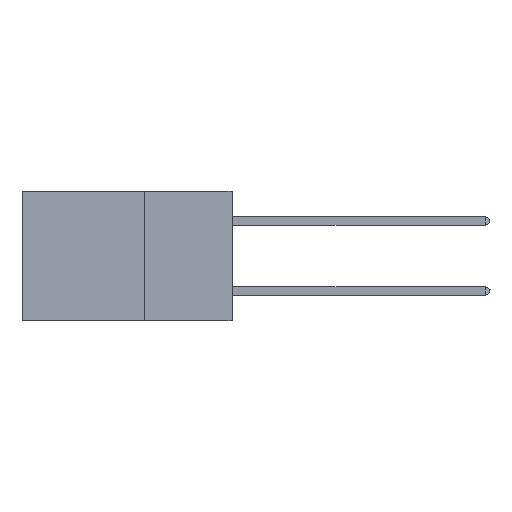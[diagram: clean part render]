
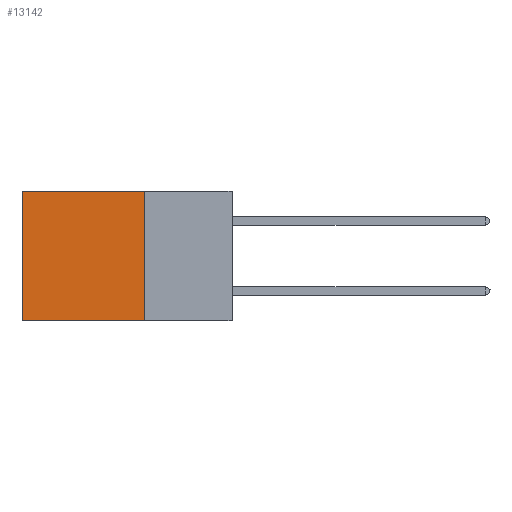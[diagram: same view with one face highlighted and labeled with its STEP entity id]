
A CAD part, left-side view. The second image highlights one B-rep face of the part: STEP entity #13142.
In plain terms, the highlighted planar face has unit normal (-1, 0, 0).
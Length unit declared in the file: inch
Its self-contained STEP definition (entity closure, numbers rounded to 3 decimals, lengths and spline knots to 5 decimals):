
#120 = CARTESIAN_POINT ( 'NONE',  ( 0.2875, 0.25, 0. ) ) ;
#332 = CARTESIAN_POINT ( 'NONE',  ( 0.2875, 0.25, -0.37 ) ) ;
#956 = ORIENTED_EDGE ( 'NONE', *, *, #16880, .F. ) ;
#1086 = VERTEX_POINT ( 'NONE', #6090 ) ;
#1681 = DIRECTION ( 'NONE',  ( 0., 1., 0. ) ) ;
#1749 = LINE ( 'NONE', #332, #8444 ) ;
#2374 = ORIENTED_EDGE ( 'NONE', *, *, #4101, .F. ) ;
#2925 = EDGE_LOOP ( 'NONE', ( #8994, #2374, #956, #4639 ) ) ;
#3289 = LINE ( 'NONE', #3307, #4132 ) ;
#3307 = CARTESIAN_POINT ( 'NONE',  ( 0.2875, 0.6, 0. ) ) ;
#3904 = PLANE ( 'NONE',  #5573 ) ;
#4068 = CARTESIAN_POINT ( 'NONE',  ( 0.2875, 0.6, 0. ) ) ;
#4101 = EDGE_CURVE ( 'NONE', #8331, #1086, #1749, .T. ) ;
#4132 = VECTOR ( 'NONE', #11289, 39.37008 ) ;
#4258 = VECTOR ( 'NONE', #8381, 39.37008 ) ;
#4639 = ORIENTED_EDGE ( 'NONE', *, *, #4806, .T. ) ;
#4806 = EDGE_CURVE ( 'NONE', #7504, #10278, #10510, .T. ) ;
#5248 = DIRECTION ( 'NONE',  ( 1., 0., 0. ) ) ;
#5573 = AXIS2_PLACEMENT_3D ( 'NONE', #13211, #5248, #14531 ) ;
#6090 = CARTESIAN_POINT ( 'NONE',  ( 0.2875, 0.6, -0.37 ) ) ;
#7504 = VERTEX_POINT ( 'NONE', #10289 ) ;
#7932 = CARTESIAN_POINT ( 'NONE',  ( 0.2875, 0.25, -0.37 ) ) ;
#8331 = VERTEX_POINT ( 'NONE', #7932 ) ;
#8381 = DIRECTION ( 'NONE',  ( 0., 1., 0. ) ) ;
#8444 = VECTOR ( 'NONE', #1681, 39.37008 ) ;
#8994 = ORIENTED_EDGE ( 'NONE', *, *, #13499, .T. ) ;
#10278 = VERTEX_POINT ( 'NONE', #4068 ) ;
#10289 = CARTESIAN_POINT ( 'NONE',  ( 0.2875, 0.25, 0. ) ) ;
#10510 = LINE ( 'NONE', #16291, #4258 ) ;
#11289 = DIRECTION ( 'NONE',  ( 0., 0., -1. ) ) ;
#12151 = DIRECTION ( 'NONE',  ( 0., 0., -1. ) ) ;
#12163 = VECTOR ( 'NONE', #12151, 39.37008 ) ;
#12274 = FACE_OUTER_BOUND ( 'NONE', #2925, .T. ) ;
#13142 = ADVANCED_FACE ( 'NONE', ( #12274 ), #3904, .F. ) ;
#13211 = CARTESIAN_POINT ( 'NONE',  ( 0.2875, 0.25, 0. ) ) ;
#13499 = EDGE_CURVE ( 'NONE', #10278, #1086, #3289, .T. ) ;
#14531 = DIRECTION ( 'NONE',  ( 0., 0., -1. ) ) ;
#15652 = LINE ( 'NONE', #120, #12163 ) ;
#16291 = CARTESIAN_POINT ( 'NONE',  ( 0.2875, 0.25, 0. ) ) ;
#16880 = EDGE_CURVE ( 'NONE', #7504, #8331, #15652, .T. ) ;
